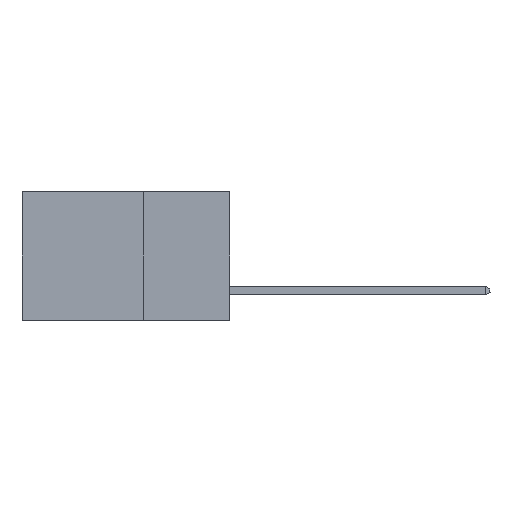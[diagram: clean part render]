
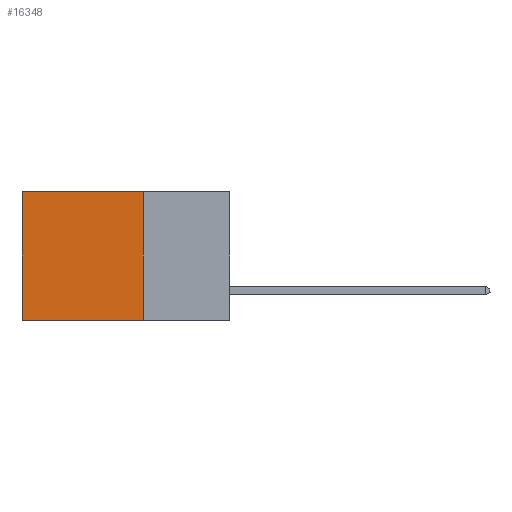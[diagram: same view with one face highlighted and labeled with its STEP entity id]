
A CAD part, left-side view. The second image highlights one B-rep face of the part: STEP entity #16348.
In plain terms, the highlighted planar face has unit normal (-1, 0, 0).
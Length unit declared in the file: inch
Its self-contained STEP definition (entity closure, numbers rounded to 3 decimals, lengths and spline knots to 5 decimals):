
#1476 = CARTESIAN_POINT ( 'NONE',  ( 0.298, 0.25, -0.37 ) ) ;
#1701 = VERTEX_POINT ( 'NONE', #7200 ) ;
#1708 = DIRECTION ( 'NONE',  ( 1., 0., 0. ) ) ;
#2355 = FACE_OUTER_BOUND ( 'NONE', #24001, .T. ) ;
#2630 = VECTOR ( 'NONE', #23938, 39.37008 ) ;
#4233 = VECTOR ( 'NONE', #12736, 39.37008 ) ;
#4250 = VECTOR ( 'NONE', #15984, 39.37008 ) ;
#4764 = EDGE_CURVE ( 'NONE', #1701, #8135, #14738, .T. ) ;
#4831 = LINE ( 'NONE', #11515, #20174 ) ;
#6726 = EDGE_CURVE ( 'NONE', #23634, #1701, #17556, .T. ) ;
#7200 = CARTESIAN_POINT ( 'NONE',  ( 0.298, 0.25, -0.37 ) ) ;
#8135 = VERTEX_POINT ( 'NONE', #11343 ) ;
#10363 = EDGE_CURVE ( 'NONE', #23634, #20629, #17243, .T. ) ;
#10689 = CARTESIAN_POINT ( 'NONE',  ( 0.298, 0.25, 0. ) ) ;
#10799 = CARTESIAN_POINT ( 'NONE',  ( 0.298, 0.25, 0. ) ) ;
#11131 = PLANE ( 'NONE',  #17860 ) ;
#11138 = ORIENTED_EDGE ( 'NONE', *, *, #4764, .F. ) ;
#11343 = CARTESIAN_POINT ( 'NONE',  ( 0.298, 0.6, -0.37 ) ) ;
#11432 = DIRECTION ( 'NONE',  ( 0., 0., -1. ) ) ;
#11515 = CARTESIAN_POINT ( 'NONE',  ( 0.298, 0.6, 0. ) ) ;
#12736 = DIRECTION ( 'NONE',  ( 0., 1., 0. ) ) ;
#13705 = ORIENTED_EDGE ( 'NONE', *, *, #6726, .F. ) ;
#14738 = LINE ( 'NONE', #1476, #2630 ) ;
#15085 = DIRECTION ( 'NONE',  ( 0., 0., -1. ) ) ;
#15983 = CARTESIAN_POINT ( 'NONE',  ( 0.298, 0.6, 0. ) ) ;
#15984 = DIRECTION ( 'NONE',  ( 0., 0., -1. ) ) ;
#16348 = ADVANCED_FACE ( 'NONE', ( #2355 ), #11131, .F. ) ;
#17243 = LINE ( 'NONE', #10799, #4233 ) ;
#17556 = LINE ( 'NONE', #21586, #4250 ) ;
#17616 = ORIENTED_EDGE ( 'NONE', *, *, #22142, .T. ) ;
#17860 = AXIS2_PLACEMENT_3D ( 'NONE', #22583, #1708, #15085 ) ;
#20174 = VECTOR ( 'NONE', #11432, 39.37008 ) ;
#20629 = VERTEX_POINT ( 'NONE', #15983 ) ;
#21266 = ORIENTED_EDGE ( 'NONE', *, *, #10363, .T. ) ;
#21586 = CARTESIAN_POINT ( 'NONE',  ( 0.298, 0.25, 0. ) ) ;
#22142 = EDGE_CURVE ( 'NONE', #20629, #8135, #4831, .T. ) ;
#22583 = CARTESIAN_POINT ( 'NONE',  ( 0.298, 0.25, 0. ) ) ;
#23634 = VERTEX_POINT ( 'NONE', #10689 ) ;
#23938 = DIRECTION ( 'NONE',  ( 0., 1., 0. ) ) ;
#24001 = EDGE_LOOP ( 'NONE', ( #17616, #11138, #13705, #21266 ) ) ;
